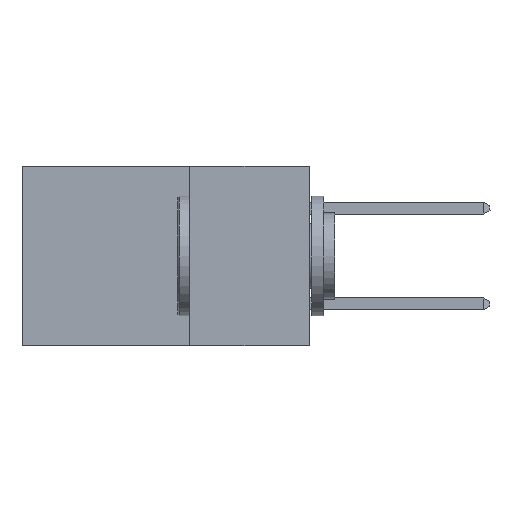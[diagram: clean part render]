
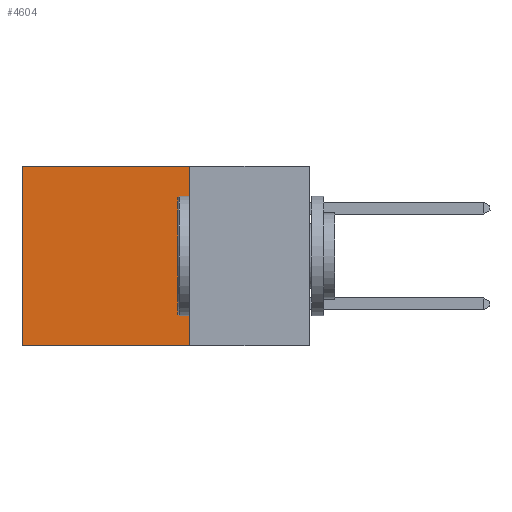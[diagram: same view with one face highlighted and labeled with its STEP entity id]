
A CAD part, left-side view. The second image highlights one B-rep face of the part: STEP entity #4604.
In plain terms, the highlighted planar face has unit normal (-1, 0, 0).
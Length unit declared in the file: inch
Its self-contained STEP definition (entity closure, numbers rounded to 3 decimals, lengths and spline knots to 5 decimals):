
#182 = CARTESIAN_POINT ( 'NONE',  ( 0.2875, 0.25, -0.375 ) ) ;
#337 = ORIENTED_EDGE ( 'NONE', *, *, #9034, .T. ) ;
#1245 = VECTOR ( 'NONE', #6189, 39.37008 ) ;
#1594 = CARTESIAN_POINT ( 'NONE',  ( 0.2875, 0.25, -0.375 ) ) ;
#1748 = VECTOR ( 'NONE', #2379, 39.37008 ) ;
#1863 = PLANE ( 'NONE',  #7045 ) ;
#1866 = CARTESIAN_POINT ( 'NONE',  ( 0.2875, 0.6, -0.375 ) ) ;
#1995 = CARTESIAN_POINT ( 'NONE',  ( 0.2875, 0.6, -0.375 ) ) ;
#2317 = LINE ( 'NONE', #5635, #9207 ) ;
#2379 = DIRECTION ( 'NONE',  ( 0., 0., -1. ) ) ;
#2552 = FACE_OUTER_BOUND ( 'NONE', #7962, .T. ) ;
#2595 = CARTESIAN_POINT ( 'NONE',  ( 0.2875, 0.6, 0. ) ) ;
#2710 = CARTESIAN_POINT ( 'NONE',  ( 0.2875, 0.25, -0.375 ) ) ;
#3145 = EDGE_CURVE ( 'NONE', #4582, #5362, #3976, .T. ) ;
#3389 = DIRECTION ( 'NONE',  ( 1., 0., 0. ) ) ;
#3548 = VECTOR ( 'NONE', #6998, 39.37008 ) ;
#3976 = LINE ( 'NONE', #1594, #1748 ) ;
#4077 = VERTEX_POINT ( 'NONE', #2595 ) ;
#4426 = ORIENTED_EDGE ( 'NONE', *, *, #3145, .F. ) ;
#4582 = VERTEX_POINT ( 'NONE', #6834 ) ;
#4604 = ADVANCED_FACE ( 'NONE', ( #2552 ), #1863, .F. ) ;
#4737 = DIRECTION ( 'NONE',  ( 0., 0., -1. ) ) ;
#4789 = CARTESIAN_POINT ( 'NONE',  ( 0.2875, 0.25, 0. ) ) ;
#4820 = EDGE_CURVE ( 'NONE', #5362, #6434, #2317, .T. ) ;
#4833 = ORIENTED_EDGE ( 'NONE', *, *, #8236, .T. ) ;
#4950 = DIRECTION ( 'NONE',  ( 0., 1., 0. ) ) ;
#5362 = VERTEX_POINT ( 'NONE', #182 ) ;
#5538 = LINE ( 'NONE', #1995, #3548 ) ;
#5635 = CARTESIAN_POINT ( 'NONE',  ( 0.2875, 0.25, -0.375 ) ) ;
#6189 = DIRECTION ( 'NONE',  ( 0., 1., 0. ) ) ;
#6230 = LINE ( 'NONE', #4789, #1245 ) ;
#6434 = VERTEX_POINT ( 'NONE', #1866 ) ;
#6495 = ORIENTED_EDGE ( 'NONE', *, *, #4820, .F. ) ;
#6834 = CARTESIAN_POINT ( 'NONE',  ( 0.2875, 0.25, 0. ) ) ;
#6998 = DIRECTION ( 'NONE',  ( 0., 0., -1. ) ) ;
#7045 = AXIS2_PLACEMENT_3D ( 'NONE', #2710, #3389, #4737 ) ;
#7962 = EDGE_LOOP ( 'NONE', ( #337, #6495, #4426, #4833 ) ) ;
#8236 = EDGE_CURVE ( 'NONE', #4582, #4077, #6230, .T. ) ;
#9034 = EDGE_CURVE ( 'NONE', #4077, #6434, #5538, .T. ) ;
#9207 = VECTOR ( 'NONE', #4950, 39.37008 ) ;
